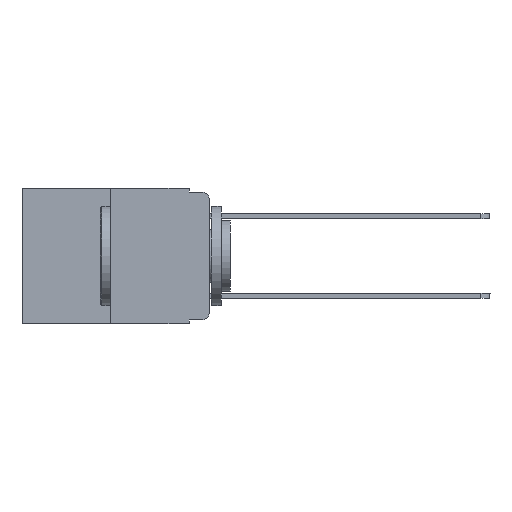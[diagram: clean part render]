
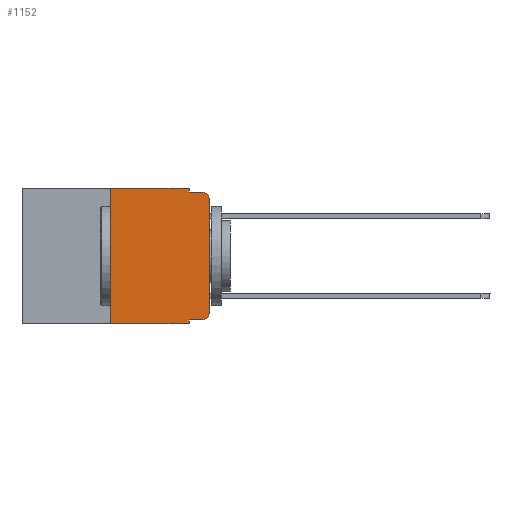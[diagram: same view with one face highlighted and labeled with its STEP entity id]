
A CAD part, left-side view. The second image highlights one B-rep face of the part: STEP entity #1152.
In plain terms, the highlighted planar face has unit normal (-1, 0, 0).
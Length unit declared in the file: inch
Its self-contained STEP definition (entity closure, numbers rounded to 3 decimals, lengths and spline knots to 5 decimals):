
#237 = EDGE_CURVE ( 'NONE', #15724, #11973, #3659, .T. ) ;
#550 = EDGE_CURVE ( 'NONE', #13799, #15724, #3597, .T. ) ;
#698 = LINE ( 'NONE', #2023, #17577 ) ;
#810 = VECTOR ( 'NONE', #8787, 39.37008 ) ;
#823 = VECTOR ( 'NONE', #2055, 39.37008 ) ;
#1152 = ADVANCED_FACE ( 'NONE', ( #7966 ), #9389, .F. ) ;
#1479 = ORIENTED_EDGE ( 'NONE', *, *, #13357, .T. ) ;
#1681 = AXIS2_PLACEMENT_3D ( 'NONE', #6839, #18059, #12551 ) ;
#2023 = CARTESIAN_POINT ( 'NONE',  ( 0., 0.473, 0. ) ) ;
#2033 = EDGE_CURVE ( 'NONE', #15590, #11973, #5545, .T. ) ;
#2055 = DIRECTION ( 'NONE',  ( 0., -1., 0. ) ) ;
#2244 = VERTEX_POINT ( 'NONE', #14531 ) ;
#2859 = DIRECTION ( 'NONE',  ( 0., 0., -1. ) ) ;
#3163 = ORIENTED_EDGE ( 'NONE', *, *, #237, .T. ) ;
#3391 = CARTESIAN_POINT ( 'NONE',  ( 0., 0.02, -0.313 ) ) ;
#3597 = LINE ( 'NONE', #17639, #9793 ) ;
#3659 = CIRCLE ( 'NONE', #13517, 0.02 ) ;
#3901 = CARTESIAN_POINT ( 'NONE',  ( 0., 0.02, -0.03 ) ) ;
#3974 = CARTESIAN_POINT ( 'NONE',  ( 0., 0.051, -0.01 ) ) ;
#4216 = VECTOR ( 'NONE', #2859, 39.37008 ) ;
#4240 = CARTESIAN_POINT ( 'NONE',  ( 0., 0.051, -0.343 ) ) ;
#5545 = LINE ( 'NONE', #3974, #14858 ) ;
#5739 = VERTEX_POINT ( 'NONE', #11196 ) ;
#5742 = LINE ( 'NONE', #11645, #4216 ) ;
#6192 = ORIENTED_EDGE ( 'NONE', *, *, #2033, .F. ) ;
#6415 = LINE ( 'NONE', #10861, #823 ) ;
#6674 = EDGE_CURVE ( 'NONE', #5739, #7869, #16138, .T. ) ;
#6839 = CARTESIAN_POINT ( 'NONE',  ( 0., 0.473, 0. ) ) ;
#7494 = AXIS2_PLACEMENT_3D ( 'NONE', #3391, #17515, #9106 ) ;
#7594 = ORIENTED_EDGE ( 'NONE', *, *, #13980, .F. ) ;
#7869 = VERTEX_POINT ( 'NONE', #14532 ) ;
#7916 = ORIENTED_EDGE ( 'NONE', *, *, #6674, .F. ) ;
#7966 = FACE_OUTER_BOUND ( 'NONE', #13615, .T. ) ;
#8010 = DIRECTION ( 'NONE',  ( 0., 0., -1. ) ) ;
#8787 = DIRECTION ( 'NONE',  ( 0., -1., 0. ) ) ;
#8998 = CARTESIAN_POINT ( 'NONE',  ( 0., 0., -0.313 ) ) ;
#9023 = DIRECTION ( 'NONE',  ( 0., 0., 1. ) ) ;
#9106 = DIRECTION ( 'NONE',  ( 0., 0., -1. ) ) ;
#9355 = EDGE_CURVE ( 'NONE', #7869, #15781, #698, .T. ) ;
#9389 = PLANE ( 'NONE',  #1681 ) ;
#9423 = LINE ( 'NONE', #15117, #9875 ) ;
#9441 = CARTESIAN_POINT ( 'NONE',  ( 0., 0.02, -0.01 ) ) ;
#9704 = DIRECTION ( 'NONE',  ( 0., 0., -1. ) ) ;
#9793 = VECTOR ( 'NONE', #14917, 39.37008 ) ;
#9875 = VECTOR ( 'NONE', #8010, 39.37008 ) ;
#10194 = CIRCLE ( 'NONE', #7494, 0.02 ) ;
#10734 = DIRECTION ( 'NONE',  ( 0., -1., 0. ) ) ;
#10861 = CARTESIAN_POINT ( 'NONE',  ( 0., 0.473, -0.343 ) ) ;
#10998 = DIRECTION ( 'NONE',  ( 0., -1., 0. ) ) ;
#11161 = VERTEX_POINT ( 'NONE', #16536 ) ;
#11196 = CARTESIAN_POINT ( 'NONE',  ( 0., 0.25, -0.343 ) ) ;
#11596 = LINE ( 'NONE', #17303, #810 ) ;
#11645 = CARTESIAN_POINT ( 'NONE',  ( 0., 0.051, 0. ) ) ;
#11973 = VERTEX_POINT ( 'NONE', #9441 ) ;
#12213 = CARTESIAN_POINT ( 'NONE',  ( 0., 0.051, -0.01 ) ) ;
#12462 = EDGE_CURVE ( 'NONE', #15781, #15590, #9423, .T. ) ;
#12530 = ORIENTED_EDGE ( 'NONE', *, *, #9355, .F. ) ;
#12551 = DIRECTION ( 'NONE',  ( 0., 0., -1. ) ) ;
#12739 = ORIENTED_EDGE ( 'NONE', *, *, #16700, .T. ) ;
#13357 = EDGE_CURVE ( 'NONE', #2244, #13799, #10194, .T. ) ;
#13517 = AXIS2_PLACEMENT_3D ( 'NONE', #3901, #18100, #9704 ) ;
#13615 = EDGE_LOOP ( 'NONE', ( #16054, #3163, #6192, #15440, #12530, #7916, #16687, #7594, #12739, #1479 ) ) ;
#13654 = VECTOR ( 'NONE', #9023, 39.37008 ) ;
#13799 = VERTEX_POINT ( 'NONE', #8998 ) ;
#13980 = EDGE_CURVE ( 'NONE', #11161, #14538, #5742, .T. ) ;
#14531 = CARTESIAN_POINT ( 'NONE',  ( 0., 0.02, -0.333 ) ) ;
#14532 = CARTESIAN_POINT ( 'NONE',  ( 0., 0.25, 0. ) ) ;
#14538 = VERTEX_POINT ( 'NONE', #4240 ) ;
#14541 = CARTESIAN_POINT ( 'NONE',  ( 0., 0.051, 0. ) ) ;
#14858 = VECTOR ( 'NONE', #10998, 39.37008 ) ;
#14917 = DIRECTION ( 'NONE',  ( 0., 0., 1. ) ) ;
#14989 = CARTESIAN_POINT ( 'NONE',  ( 0., 0.25, 0. ) ) ;
#15117 = CARTESIAN_POINT ( 'NONE',  ( 0., 0.051, 0. ) ) ;
#15440 = ORIENTED_EDGE ( 'NONE', *, *, #12462, .F. ) ;
#15590 = VERTEX_POINT ( 'NONE', #12213 ) ;
#15668 = CARTESIAN_POINT ( 'NONE',  ( 0., 0., -0.03 ) ) ;
#15724 = VERTEX_POINT ( 'NONE', #15668 ) ;
#15781 = VERTEX_POINT ( 'NONE', #14541 ) ;
#16054 = ORIENTED_EDGE ( 'NONE', *, *, #550, .T. ) ;
#16138 = LINE ( 'NONE', #14989, #13654 ) ;
#16536 = CARTESIAN_POINT ( 'NONE',  ( 0., 0.051, -0.333 ) ) ;
#16687 = ORIENTED_EDGE ( 'NONE', *, *, #16813, .T. ) ;
#16700 = EDGE_CURVE ( 'NONE', #11161, #2244, #11596, .T. ) ;
#16813 = EDGE_CURVE ( 'NONE', #5739, #14538, #6415, .T. ) ;
#17303 = CARTESIAN_POINT ( 'NONE',  ( 0., 0.051, -0.333 ) ) ;
#17515 = DIRECTION ( 'NONE',  ( -1., 0., 0. ) ) ;
#17577 = VECTOR ( 'NONE', #10734, 39.37008 ) ;
#17639 = CARTESIAN_POINT ( 'NONE',  ( 0., 0., 0. ) ) ;
#18059 = DIRECTION ( 'NONE',  ( 1., 0., 0. ) ) ;
#18100 = DIRECTION ( 'NONE',  ( -1., 0., 0. ) ) ;
